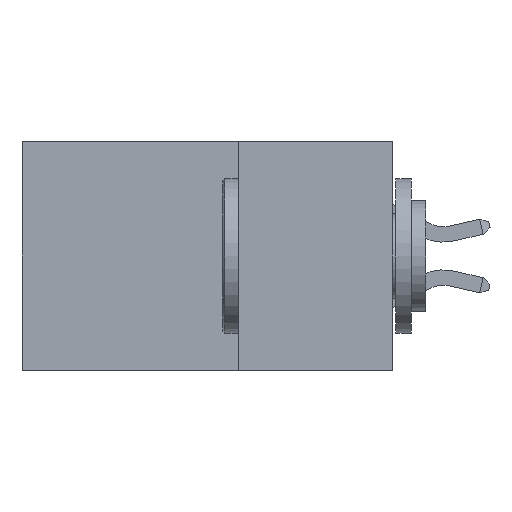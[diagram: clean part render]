
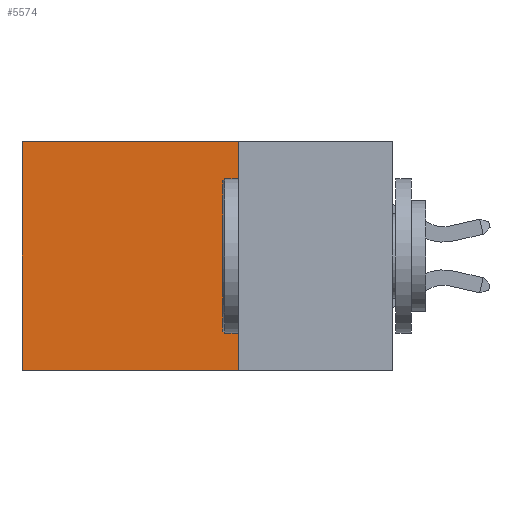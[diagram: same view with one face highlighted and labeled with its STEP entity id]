
A CAD part, left-side view. The second image highlights one B-rep face of the part: STEP entity #5574.
In plain terms, the highlighted planar face has unit normal (-1, 0, 0).
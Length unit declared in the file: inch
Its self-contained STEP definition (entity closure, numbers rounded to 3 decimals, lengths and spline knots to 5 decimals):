
#1036 = VERTEX_POINT ( 'NONE', #21527 ) ;
#1349 = CARTESIAN_POINT ( 'NONE',  ( 0.2875, 0.25, 0. ) ) ;
#2775 = CARTESIAN_POINT ( 'NONE',  ( 0.2875, 0.25, -0.37 ) ) ;
#3270 = DIRECTION ( 'NONE',  ( 1., 0., 0. ) ) ;
#3307 = VERTEX_POINT ( 'NONE', #2775 ) ;
#3953 = DIRECTION ( 'NONE',  ( 0., 0., -1. ) ) ;
#4248 = VECTOR ( 'NONE', #20436, 39.37008 ) ;
#5526 = VECTOR ( 'NONE', #18090, 39.37008 ) ;
#5574 = ADVANCED_FACE ( 'NONE', ( #9949 ), #10381, .F. ) ;
#5709 = EDGE_CURVE ( 'NONE', #1036, #16880, #17850, .T. ) ;
#5765 = ORIENTED_EDGE ( 'NONE', *, *, #6239, .F. ) ;
#5954 = LINE ( 'NONE', #20657, #4248 ) ;
#6239 = EDGE_CURVE ( 'NONE', #3307, #10513, #5954, .T. ) ;
#7052 = CARTESIAN_POINT ( 'NONE',  ( 0.2875, 0.6, -0.37 ) ) ;
#7091 = DIRECTION ( 'NONE',  ( 0., 1., 0. ) ) ;
#8166 = VECTOR ( 'NONE', #3953, 39.37008 ) ;
#9024 = EDGE_LOOP ( 'NONE', ( #10040, #5765, #18536, #18972 ) ) ;
#9949 = FACE_OUTER_BOUND ( 'NONE', #9024, .T. ) ;
#10040 = ORIENTED_EDGE ( 'NONE', *, *, #23186, .T. ) ;
#10381 = PLANE ( 'NONE',  #13400 ) ;
#10467 = CARTESIAN_POINT ( 'NONE',  ( 0.2875, 0.6, 0. ) ) ;
#10513 = VERTEX_POINT ( 'NONE', #7052 ) ;
#10735 = LINE ( 'NONE', #12893, #8166 ) ;
#12893 = CARTESIAN_POINT ( 'NONE',  ( 0.2875, 0.6, 0. ) ) ;
#13163 = EDGE_CURVE ( 'NONE', #1036, #3307, #18841, .T. ) ;
#13400 = AXIS2_PLACEMENT_3D ( 'NONE', #17568, #3270, #13765 ) ;
#13765 = DIRECTION ( 'NONE',  ( 0., 0., -1. ) ) ;
#14394 = CARTESIAN_POINT ( 'NONE',  ( 0.2875, 0.25, 0. ) ) ;
#16143 = VECTOR ( 'NONE', #7091, 39.37008 ) ;
#16880 = VERTEX_POINT ( 'NONE', #10467 ) ;
#17568 = CARTESIAN_POINT ( 'NONE',  ( 0.2875, 0.25, 0. ) ) ;
#17850 = LINE ( 'NONE', #14394, #16143 ) ;
#18090 = DIRECTION ( 'NONE',  ( 0., 0., -1. ) ) ;
#18536 = ORIENTED_EDGE ( 'NONE', *, *, #13163, .F. ) ;
#18841 = LINE ( 'NONE', #1349, #5526 ) ;
#18972 = ORIENTED_EDGE ( 'NONE', *, *, #5709, .T. ) ;
#20436 = DIRECTION ( 'NONE',  ( 0., 1., 0. ) ) ;
#20657 = CARTESIAN_POINT ( 'NONE',  ( 0.2875, 0.25, -0.37 ) ) ;
#21527 = CARTESIAN_POINT ( 'NONE',  ( 0.2875, 0.25, 0. ) ) ;
#23186 = EDGE_CURVE ( 'NONE', #16880, #10513, #10735, .T. ) ;
